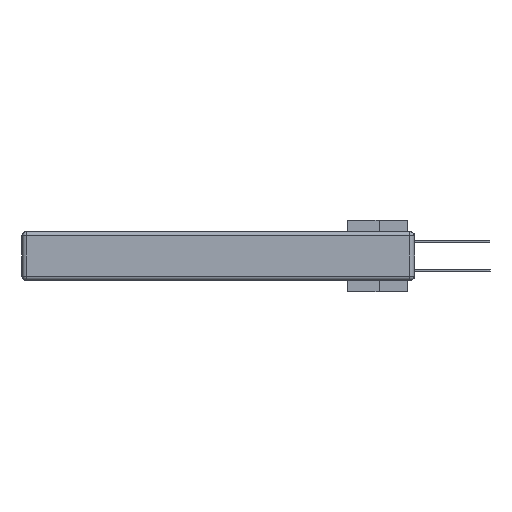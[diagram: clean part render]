
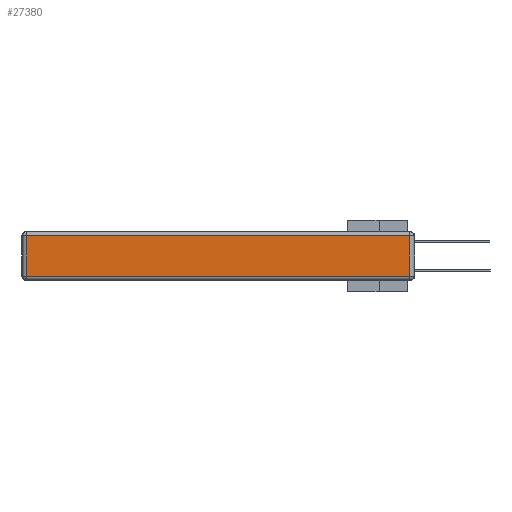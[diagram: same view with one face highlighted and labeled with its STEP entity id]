
A CAD part, left-side view. The second image highlights one B-rep face of the part: STEP entity #27380.
In plain terms, the highlighted planar face has unit normal (-1, 0, 0).
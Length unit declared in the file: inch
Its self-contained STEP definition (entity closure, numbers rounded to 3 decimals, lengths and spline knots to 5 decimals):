
#1418 = VERTEX_POINT ( 'NONE', #18375 ) ;
#1435 = CARTESIAN_POINT ( 'NONE',  ( 0., 2.72, -0.03 ) ) ;
#2054 = CARTESIAN_POINT ( 'NONE',  ( 0., 2.72, -0.343 ) ) ;
#4009 = VECTOR ( 'NONE', #10945, 39.37008 ) ;
#4807 = FACE_OUTER_BOUND ( 'NONE', #27859, .T. ) ;
#5626 = LINE ( 'NONE', #2054, #16619 ) ;
#6164 = CARTESIAN_POINT ( 'NONE',  ( 0., 0.03, -0.343 ) ) ;
#10525 = LINE ( 'NONE', #20203, #4009 ) ;
#10945 = DIRECTION ( 'NONE',  ( 0., -1., 0. ) ) ;
#11591 = CARTESIAN_POINT ( 'NONE',  ( 0., 0.03, -0.313 ) ) ;
#11760 = VERTEX_POINT ( 'NONE', #17383 ) ;
#13647 = ORIENTED_EDGE ( 'NONE', *, *, #25112, .T. ) ;
#13955 = VERTEX_POINT ( 'NONE', #11591 ) ;
#14726 = CARTESIAN_POINT ( 'NONE',  ( 0., 0., -0.343 ) ) ;
#14913 = DIRECTION ( 'NONE',  ( 0., 0., -1. ) ) ;
#15343 = LINE ( 'NONE', #21667, #27753 ) ;
#16619 = VECTOR ( 'NONE', #14913, 39.37008 ) ;
#17383 = CARTESIAN_POINT ( 'NONE',  ( 0., 0.03, -0.03 ) ) ;
#18296 = AXIS2_PLACEMENT_3D ( 'NONE', #14726, #24219, #26744 ) ;
#18375 = CARTESIAN_POINT ( 'NONE',  ( 0., 2.72, -0.313 ) ) ;
#19020 = DIRECTION ( 'NONE',  ( 0., 0., 1. ) ) ;
#20203 = CARTESIAN_POINT ( 'NONE',  ( 0., 0., -0.313 ) ) ;
#20356 = ORIENTED_EDGE ( 'NONE', *, *, #36515, .T. ) ;
#21667 = CARTESIAN_POINT ( 'NONE',  ( 0., 2.75, -0.03 ) ) ;
#24219 = DIRECTION ( 'NONE',  ( -1., 0., 0. ) ) ;
#25112 = EDGE_CURVE ( 'NONE', #1418, #13955, #10525, .T. ) ;
#26744 = DIRECTION ( 'NONE',  ( 0., 0., 1. ) ) ;
#27380 = ADVANCED_FACE ( 'NONE', ( #4807 ), #36410, .T. ) ;
#27410 = VERTEX_POINT ( 'NONE', #1435 ) ;
#27590 = EDGE_CURVE ( 'NONE', #11760, #27410, #15343, .T. ) ;
#27753 = VECTOR ( 'NONE', #40836, 39.37008 ) ;
#27859 = EDGE_LOOP ( 'NONE', ( #13647, #35579, #31940, #20356 ) ) ;
#28725 = LINE ( 'NONE', #6164, #41192 ) ;
#31288 = EDGE_CURVE ( 'NONE', #13955, #11760, #28725, .T. ) ;
#31940 = ORIENTED_EDGE ( 'NONE', *, *, #27590, .T. ) ;
#35579 = ORIENTED_EDGE ( 'NONE', *, *, #31288, .T. ) ;
#36410 = PLANE ( 'NONE',  #18296 ) ;
#36515 = EDGE_CURVE ( 'NONE', #27410, #1418, #5626, .T. ) ;
#40836 = DIRECTION ( 'NONE',  ( 0., 1., 0. ) ) ;
#41192 = VECTOR ( 'NONE', #19020, 39.37008 ) ;
